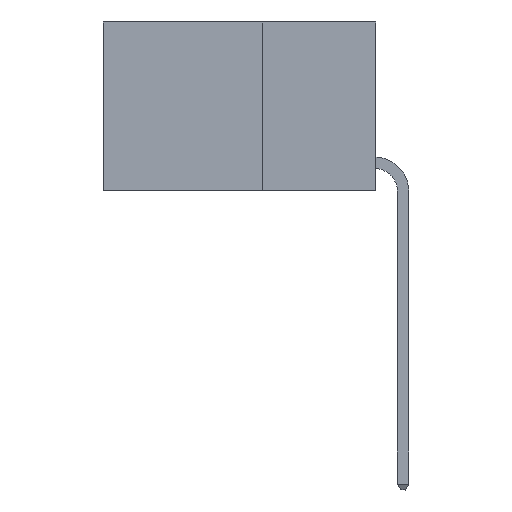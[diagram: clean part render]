
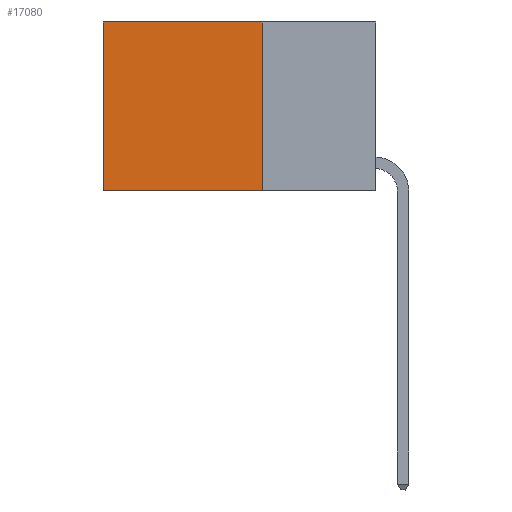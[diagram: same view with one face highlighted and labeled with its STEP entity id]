
A CAD part, left-side view. The second image highlights one B-rep face of the part: STEP entity #17080.
In plain terms, the highlighted planar face has unit normal (-1, 0, 0).
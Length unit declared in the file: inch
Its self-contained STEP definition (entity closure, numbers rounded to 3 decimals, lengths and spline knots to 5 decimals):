
#406 = CARTESIAN_POINT ( 'NONE',  ( 0.2625, 0.25, 0. ) ) ;
#531 = CARTESIAN_POINT ( 'NONE',  ( 0.2625, 0.6, 0. ) ) ;
#1088 = VERTEX_POINT ( 'NONE', #17173 ) ;
#1786 = VECTOR ( 'NONE', #16073, 39.37008 ) ;
#2215 = ORIENTED_EDGE ( 'NONE', *, *, #18610, .F. ) ;
#2295 = VERTEX_POINT ( 'NONE', #19560 ) ;
#2357 = FACE_OUTER_BOUND ( 'NONE', #19953, .T. ) ;
#3638 = AXIS2_PLACEMENT_3D ( 'NONE', #3644, #14629, #5227 ) ;
#3644 = CARTESIAN_POINT ( 'NONE',  ( 0.2625, 0.25, 0. ) ) ;
#5227 = DIRECTION ( 'NONE',  ( 0., 0., -1. ) ) ;
#7252 = CARTESIAN_POINT ( 'NONE',  ( 0.2625, 0.25, 0. ) ) ;
#8942 = EDGE_CURVE ( 'NONE', #1088, #2295, #13627, .T. ) ;
#9039 = ORIENTED_EDGE ( 'NONE', *, *, #9463, .T. ) ;
#9248 = LINE ( 'NONE', #406, #1786 ) ;
#9276 = LINE ( 'NONE', #19745, #13432 ) ;
#9406 = EDGE_CURVE ( 'NONE', #1088, #14416, #9248, .T. ) ;
#9463 = EDGE_CURVE ( 'NONE', #14416, #13824, #20123, .T. ) ;
#10502 = DIRECTION ( 'NONE',  ( 0., 1., 0. ) ) ;
#11195 = ORIENTED_EDGE ( 'NONE', *, *, #9406, .T. ) ;
#11684 = CARTESIAN_POINT ( 'NONE',  ( 0.2625, 0.6, 0. ) ) ;
#12201 = ORIENTED_EDGE ( 'NONE', *, *, #8942, .F. ) ;
#13432 = VECTOR ( 'NONE', #10502, 39.37008 ) ;
#13627 = LINE ( 'NONE', #7252, #17235 ) ;
#13824 = VERTEX_POINT ( 'NONE', #17878 ) ;
#14416 = VERTEX_POINT ( 'NONE', #531 ) ;
#14629 = DIRECTION ( 'NONE',  ( 1., 0., 0. ) ) ;
#14801 = DIRECTION ( 'NONE',  ( 0., 0., -1. ) ) ;
#16073 = DIRECTION ( 'NONE',  ( 0., 1., 0. ) ) ;
#16542 = VECTOR ( 'NONE', #14801, 39.37008 ) ;
#17080 = ADVANCED_FACE ( 'NONE', ( #2357 ), #19197, .F. ) ;
#17173 = CARTESIAN_POINT ( 'NONE',  ( 0.2625, 0.25, 0. ) ) ;
#17235 = VECTOR ( 'NONE', #19713, 39.37008 ) ;
#17878 = CARTESIAN_POINT ( 'NONE',  ( 0.2625, 0.6, -0.37 ) ) ;
#18610 = EDGE_CURVE ( 'NONE', #2295, #13824, #9276, .T. ) ;
#19197 = PLANE ( 'NONE',  #3638 ) ;
#19560 = CARTESIAN_POINT ( 'NONE',  ( 0.2625, 0.25, -0.37 ) ) ;
#19713 = DIRECTION ( 'NONE',  ( 0., 0., -1. ) ) ;
#19745 = CARTESIAN_POINT ( 'NONE',  ( 0.2625, 0.25, -0.37 ) ) ;
#19953 = EDGE_LOOP ( 'NONE', ( #9039, #2215, #12201, #11195 ) ) ;
#20123 = LINE ( 'NONE', #11684, #16542 ) ;
